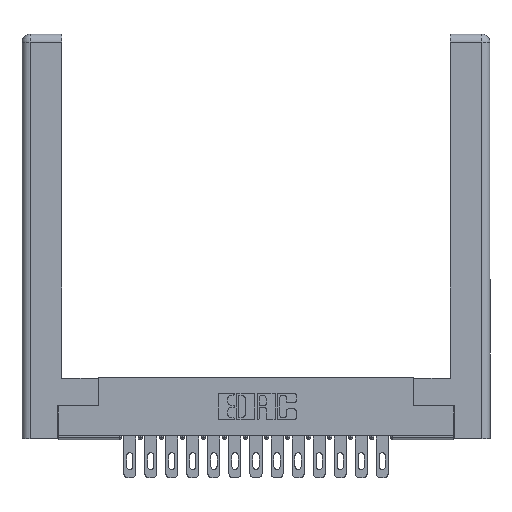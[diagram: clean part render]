
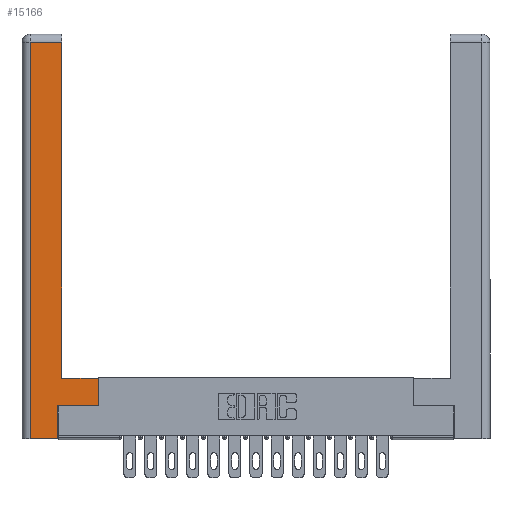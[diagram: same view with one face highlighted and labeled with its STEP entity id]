
A CAD part, top view. The second image highlights one B-rep face of the part: STEP entity #15166.
In plain terms, the highlighted planar face has unit normal (0, 0, 1).
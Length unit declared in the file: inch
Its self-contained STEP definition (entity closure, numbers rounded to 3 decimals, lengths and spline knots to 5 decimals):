
#1423 = VECTOR ( 'NONE', #1533, 39.37008 ) ;
#1521 = VECTOR ( 'NONE', #2165, 39.37008 ) ;
#1533 = DIRECTION ( 'NONE',  ( 1., 0., 0. ) ) ;
#2165 = DIRECTION ( 'NONE',  ( 0., 1., 0. ) ) ;
#2754 = EDGE_CURVE ( 'NONE', #15740, #9194, #9987, .T. ) ;
#3165 = ORIENTED_EDGE ( 'NONE', *, *, #16483, .T. ) ;
#3316 = CARTESIAN_POINT ( 'NONE',  ( 0.265, 0.245, 0. ) ) ;
#3449 = DIRECTION ( 'NONE',  ( 0., 1., 0. ) ) ;
#3456 = ORIENTED_EDGE ( 'NONE', *, *, #9795, .T. ) ;
#3732 = VERTEX_POINT ( 'NONE', #3316 ) ;
#3745 = EDGE_CURVE ( 'NONE', #14284, #19712, #18463, .T. ) ;
#3750 = CARTESIAN_POINT ( 'NONE',  ( 0.265, 0., 0. ) ) ;
#3949 = CARTESIAN_POINT ( 'NONE',  ( 0.265, 0., 0. ) ) ;
#4421 = DIRECTION ( 'NONE',  ( -1., 0., 0. ) ) ;
#5082 = LINE ( 'NONE', #7837, #1423 ) ;
#5454 = DIRECTION ( 'NONE',  ( -1., 0., 0. ) ) ;
#5728 = DIRECTION ( 'NONE',  ( 0., 0., -1. ) ) ;
#6050 = CARTESIAN_POINT ( 'NONE',  ( 0.265, 0.245, 0. ) ) ;
#6179 = LINE ( 'NONE', #3949, #10619 ) ;
#6295 = VECTOR ( 'NONE', #4421, 39.37008 ) ;
#6403 = LINE ( 'NONE', #17825, #1521 ) ;
#7000 = VECTOR ( 'NONE', #12229, 39.37008 ) ;
#7120 = CARTESIAN_POINT ( 'NONE',  ( 0.565, 0.45, 0. ) ) ;
#7419 = EDGE_CURVE ( 'NONE', #11401, #3732, #8826, .T. ) ;
#7837 = CARTESIAN_POINT ( 'NONE',  ( 0.565, 0.245, 0. ) ) ;
#7998 = VECTOR ( 'NONE', #3449, 39.37008 ) ;
#8042 = DIRECTION ( 'NONE',  ( 0., -1., 0. ) ) ;
#8826 = LINE ( 'NONE', #6050, #12986 ) ;
#9101 = AXIS2_PLACEMENT_3D ( 'NONE', #18048, #5728, #5454 ) ;
#9194 = VERTEX_POINT ( 'NONE', #14654 ) ;
#9795 = EDGE_CURVE ( 'NONE', #19712, #11401, #6179, .T. ) ;
#9803 = EDGE_CURVE ( 'NONE', #12617, #15740, #6403, .T. ) ;
#9987 = LINE ( 'NONE', #16846, #7000 ) ;
#10184 = ORIENTED_EDGE ( 'NONE', *, *, #9803, .T. ) ;
#10442 = ORIENTED_EDGE ( 'NONE', *, *, #3745, .T. ) ;
#10619 = VECTOR ( 'NONE', #13283, 39.37008 ) ;
#10945 = LINE ( 'NONE', #14271, #7998 ) ;
#10999 = CARTESIAN_POINT ( 'NONE',  ( 0.295, 2.94, 0. ) ) ;
#11401 = VERTEX_POINT ( 'NONE', #3750 ) ;
#12229 = DIRECTION ( 'NONE',  ( -1., 0., 0. ) ) ;
#12487 = EDGE_LOOP ( 'NONE', ( #12647, #19765, #10442, #3456, #14071, #3165, #10184, #14101 ) ) ;
#12617 = VERTEX_POINT ( 'NONE', #19611 ) ;
#12647 = ORIENTED_EDGE ( 'NONE', *, *, #13394, .T. ) ;
#12986 = VECTOR ( 'NONE', #13805, 39.37008 ) ;
#13283 = DIRECTION ( 'NONE',  ( 1., 0., 0. ) ) ;
#13294 = PLANE ( 'NONE',  #9101 ) ;
#13394 = EDGE_CURVE ( 'NONE', #9194, #16434, #10945, .T. ) ;
#13805 = DIRECTION ( 'NONE',  ( 0., 1., 0. ) ) ;
#14071 = ORIENTED_EDGE ( 'NONE', *, *, #7419, .T. ) ;
#14101 = ORIENTED_EDGE ( 'NONE', *, *, #2754, .T. ) ;
#14271 = CARTESIAN_POINT ( 'NONE',  ( 0.295, 3., 0. ) ) ;
#14284 = VERTEX_POINT ( 'NONE', #15520 ) ;
#14654 = CARTESIAN_POINT ( 'NONE',  ( 0.295, 0.45, 0. ) ) ;
#15166 = ADVANCED_FACE ( 'NONE', ( #20079 ), #13294, .F. ) ;
#15245 = CARTESIAN_POINT ( 'NONE',  ( 0.0615, 2.94, 0. ) ) ;
#15520 = CARTESIAN_POINT ( 'NONE',  ( 0.0615, 2.94, 0. ) ) ;
#15740 = VERTEX_POINT ( 'NONE', #7120 ) ;
#15770 = CARTESIAN_POINT ( 'NONE',  ( 0.0615, 0., 0. ) ) ;
#16274 = VECTOR ( 'NONE', #8042, 39.37008 ) ;
#16372 = CARTESIAN_POINT ( 'NONE',  ( 0.0615, 0., 0. ) ) ;
#16434 = VERTEX_POINT ( 'NONE', #10999 ) ;
#16483 = EDGE_CURVE ( 'NONE', #3732, #12617, #5082, .T. ) ;
#16846 = CARTESIAN_POINT ( 'NONE',  ( 0.295, 0.45, 0. ) ) ;
#17088 = EDGE_CURVE ( 'NONE', #16434, #14284, #19752, .T. ) ;
#17825 = CARTESIAN_POINT ( 'NONE',  ( 0.565, 0.45, 0. ) ) ;
#18048 = CARTESIAN_POINT ( 'NONE',  ( 0., 0., 0. ) ) ;
#18463 = LINE ( 'NONE', #15770, #16274 ) ;
#19611 = CARTESIAN_POINT ( 'NONE',  ( 0.565, 0.245, 0. ) ) ;
#19712 = VERTEX_POINT ( 'NONE', #16372 ) ;
#19752 = LINE ( 'NONE', #15245, #6295 ) ;
#19765 = ORIENTED_EDGE ( 'NONE', *, *, #17088, .T. ) ;
#20079 = FACE_OUTER_BOUND ( 'NONE', #12487, .T. ) ;
